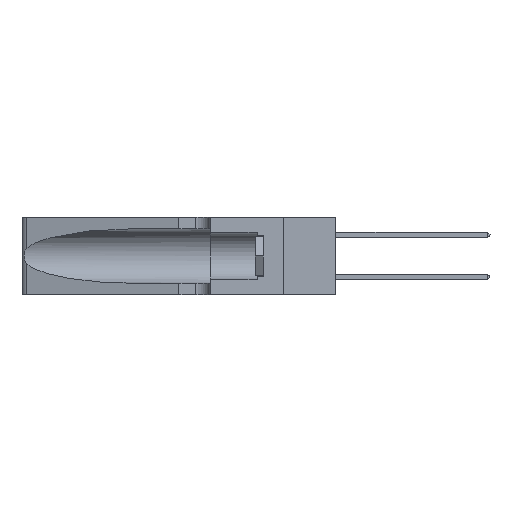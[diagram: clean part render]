
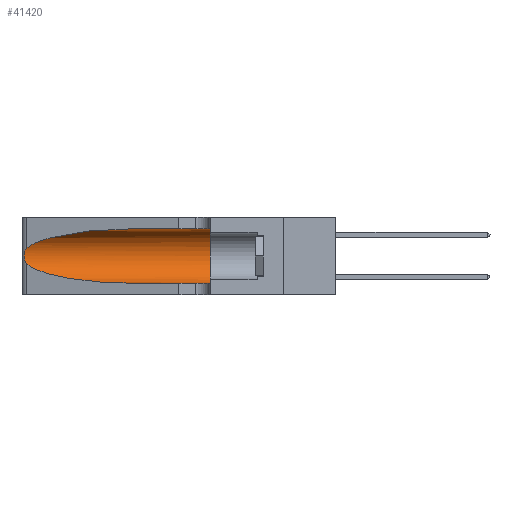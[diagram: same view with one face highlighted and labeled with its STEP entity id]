
A CAD part, left-side view. The second image highlights one B-rep face of the part: STEP entity #41420.
In plain terms, the highlighted cylindrical face has radius 3.308 mm (diameter 6.617 mm), a partial arc.
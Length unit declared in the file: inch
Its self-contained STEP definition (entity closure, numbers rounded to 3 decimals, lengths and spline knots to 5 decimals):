
#1022 = CARTESIAN_POINT ( 'NONE',  ( 0.25787, 1.23484, 0.2124 ) ) ;
#1656 = CARTESIAN_POINT ( 'NONE',  ( 0.25487, 1.22718, 0.14631 ) ) ;
#2105 = CARTESIAN_POINT ( 'NONE',  ( 0.25555, 1.22993, 0.14849 ) ) ;
#3797 = CARTESIAN_POINT ( 'NONE',  ( 0.25487, 1.22718, 0.14631 ) ) ;
#4090 = CARTESIAN_POINT ( 'NONE',  ( 0.1305, 0.35, 0.05475 ) ) ;
#4092 = ORIENTED_EDGE ( 'NONE', *, *, #39952, .T. ) ;
#4315 = CARTESIAN_POINT ( 'NONE',  ( 0.25487, 1.22718, 0.22369 ) ) ;
#8078 = CARTESIAN_POINT ( 'NONE',  ( 0.1305, 1.61858, 0.05475 ) ) ;
#8442 = VERTEX_POINT ( 'NONE', #31095 ) ;
#8569 =( BOUNDED_CURVE ( )  B_SPLINE_CURVE ( 3, ( #30251, #19621, #42270, #13311 ),
 .UNSPECIFIED., .F., .F. ) 
 B_SPLINE_CURVE_WITH_KNOTS ( ( 4, 4 ),
 ( 3.44316, 4.71239 ),
 .UNSPECIFIED. ) 
 CURVE ( )  GEOMETRIC_REPRESENTATION_ITEM ( )  RATIONAL_B_SPLINE_CURVE ( ( 1., 0.87, 0.87, 1. ) ) 
 REPRESENTATION_ITEM ( '' )  );
#10070 = VERTEX_POINT ( 'NONE', #3797 ) ;
#11317 = VERTEX_POINT ( 'NONE', #18476 ) ;
#11476 = EDGE_CURVE ( 'NONE', #23600, #8442, #46034, .T. ) ;
#12541 = ORIENTED_EDGE ( 'NONE', *, *, #13510, .T. ) ;
#12653 = CARTESIAN_POINT ( 'NONE',  ( 0.25856, 1.23593, 0.16098 ) ) ;
#13289 = DIRECTION ( 'NONE',  ( 0., 0., 1. ) ) ;
#13311 = CARTESIAN_POINT ( 'NONE',  ( 0.1305, 0.72297, 0.05475 ) ) ;
#13443 = B_SPLINE_CURVE_WITH_KNOTS ( 'NONE', 3,
 ( #4315, #36914, #18975, #1022, #30670, #30816, #16449, #27313, #34409, #12653, #33959, #27007, #2105, #1656 ),
 .UNSPECIFIED., .F., .F.,
 ( 4, 2, 2, 2, 2, 2, 4 ),
 ( 0., 0.00027, 0.00053, 0.00107, 0.0016, 0.00187, 0.00214 ),
 .UNSPECIFIED. ) ;
#13504 = AXIS2_PLACEMENT_3D ( 'NONE', #38988, #24515, #38680 ) ;
#13510 = EDGE_CURVE ( 'NONE', #23600, #23103, #34280, .T. ) ;
#16449 = CARTESIAN_POINT ( 'NONE',  ( 0.26075, 1.23896, 0.19203 ) ) ;
#18459 = DIRECTION ( 'NONE',  ( 0., -1., 0. ) ) ;
#18476 = CARTESIAN_POINT ( 'NONE',  ( 0.1305, 0.72297, 0.05475 ) ) ;
#18975 = CARTESIAN_POINT ( 'NONE',  ( 0.25639, 1.23184, 0.21858 ) ) ;
#19621 = CARTESIAN_POINT ( 'NONE',  ( 0.2373, 1.15595, 0.08982 ) ) ;
#20363 = DIRECTION ( 'NONE',  ( 0., 1., 0. ) ) ;
#21273 = CARTESIAN_POINT ( 'NONE',  ( 0.1305, 0.72297, 0.31525 ) ) ;
#23103 = VERTEX_POINT ( 'NONE', #28724 ) ;
#23600 = VERTEX_POINT ( 'NONE', #35267 ) ;
#23877 = AXIS2_PLACEMENT_3D ( 'NONE', #27635, #20363, #13289 ) ;
#24515 = DIRECTION ( 'NONE',  ( 0., -1., 0. ) ) ;
#27007 = CARTESIAN_POINT ( 'NONE',  ( 0.25639, 1.23186, 0.15144 ) ) ;
#27313 = CARTESIAN_POINT ( 'NONE',  ( 0.26075, 1.23896, 0.178 ) ) ;
#27635 = CARTESIAN_POINT ( 'NONE',  ( 0.1305, 0.35, 0.185 ) ) ;
#28498 = LINE ( 'NONE', #8078, #33030 ) ;
#28563 = VECTOR ( 'NONE', #35307, 39.37008 ) ;
#28724 = CARTESIAN_POINT ( 'NONE',  ( 0.25487, 1.22718, 0.22369 ) ) ;
#28731 = CARTESIAN_POINT ( 'NONE',  ( 0.1305, 1.61858, 0.31525 ) ) ;
#28741 = CARTESIAN_POINT ( 'NONE',  ( 0.2373, 1.15595, 0.28018 ) ) ;
#30251 = CARTESIAN_POINT ( 'NONE',  ( 0.25487, 1.22718, 0.14631 ) ) ;
#30670 = CARTESIAN_POINT ( 'NONE',  ( 0.25854, 1.2359, 0.20912 ) ) ;
#30816 = CARTESIAN_POINT ( 'NONE',  ( 0.26018, 1.23835, 0.19895 ) ) ;
#31095 = CARTESIAN_POINT ( 'NONE',  ( 0.1305, 0.35, 0.31525 ) ) ;
#32053 = EDGE_CURVE ( 'NONE', #8442, #35676, #38006, .T. ) ;
#32828 = CARTESIAN_POINT ( 'NONE',  ( 0.25487, 1.22718, 0.22369 ) ) ;
#33030 = VECTOR ( 'NONE', #18459, 39.37008 ) ;
#33286 = ORIENTED_EDGE ( 'NONE', *, *, #38196, .T. ) ;
#33959 = CARTESIAN_POINT ( 'NONE',  ( 0.25789, 1.23486, 0.15765 ) ) ;
#34280 =( BOUNDED_CURVE ( )  B_SPLINE_CURVE ( 3, ( #21273, #38521, #28741, #32828 ),
 .UNSPECIFIED., .F., .T. ) 
 B_SPLINE_CURVE_WITH_KNOTS ( ( 4, 4 ),
 ( 1.5708, 2.84003 ),
 .UNSPECIFIED. ) 
 CURVE ( )  GEOMETRIC_REPRESENTATION_ITEM ( )  RATIONAL_B_SPLINE_CURVE ( ( 1., 0.87, 0.87, 1. ) ) 
 REPRESENTATION_ITEM ( '' )  );
#34409 = CARTESIAN_POINT ( 'NONE',  ( 0.26017, 1.23833, 0.17102 ) ) ;
#35267 = CARTESIAN_POINT ( 'NONE',  ( 0.1305, 0.72297, 0.31525 ) ) ;
#35307 = DIRECTION ( 'NONE',  ( 0., -1., 0. ) ) ;
#35676 = VERTEX_POINT ( 'NONE', #4090 ) ;
#36914 = CARTESIAN_POINT ( 'NONE',  ( 0.25555, 1.22994, 0.2215 ) ) ;
#38006 = CIRCLE ( 'NONE', #23877, 0.13025 ) ;
#38196 = EDGE_CURVE ( 'NONE', #11317, #35676, #28498, .T. ) ;
#38216 = FACE_OUTER_BOUND ( 'NONE', #42552, .T. ) ;
#38521 = CARTESIAN_POINT ( 'NONE',  ( 0.18966, 0.96281, 0.31525 ) ) ;
#38680 = DIRECTION ( 'NONE',  ( 0., 0., -1. ) ) ;
#38988 = CARTESIAN_POINT ( 'NONE',  ( 0.1305, 1.61858, 0.185 ) ) ;
#39690 = EDGE_CURVE ( 'NONE', #23103, #10070, #13443, .T. ) ;
#39952 = EDGE_CURVE ( 'NONE', #10070, #11317, #8569, .T. ) ;
#41033 = CYLINDRICAL_SURFACE ( 'NONE', #13504, 0.13025 ) ;
#41420 = ADVANCED_FACE ( 'NONE', ( #38216 ), #41033, .F. ) ;
#42263 = ORIENTED_EDGE ( 'NONE', *, *, #11476, .F. ) ;
#42270 = CARTESIAN_POINT ( 'NONE',  ( 0.18966, 0.96281, 0.05475 ) ) ;
#42552 = EDGE_LOOP ( 'NONE', ( #12541, #45977, #4092, #33286, #45121, #42263 ) ) ;
#45121 = ORIENTED_EDGE ( 'NONE', *, *, #32053, .F. ) ;
#45977 = ORIENTED_EDGE ( 'NONE', *, *, #39690, .T. ) ;
#46034 = LINE ( 'NONE', #28731, #28563 ) ;
